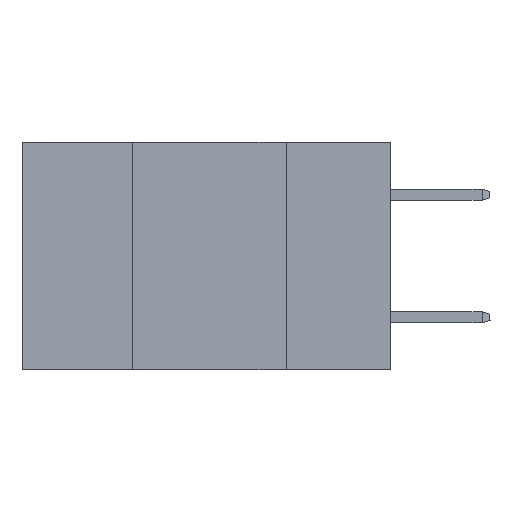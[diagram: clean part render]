
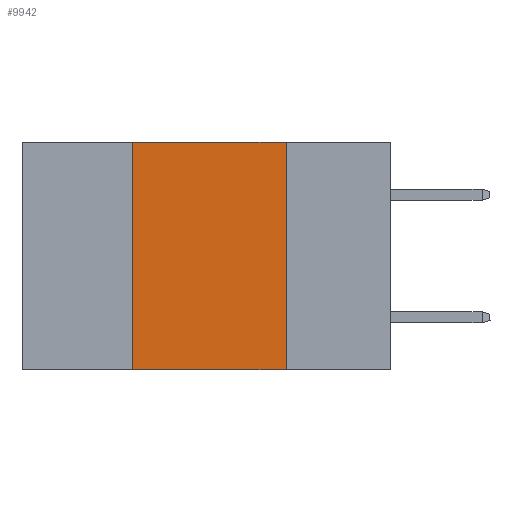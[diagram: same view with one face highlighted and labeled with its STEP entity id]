
A CAD part, left-side view. The second image highlights one B-rep face of the part: STEP entity #9942.
In plain terms, the highlighted planar face has unit normal (-1, 0, 0).
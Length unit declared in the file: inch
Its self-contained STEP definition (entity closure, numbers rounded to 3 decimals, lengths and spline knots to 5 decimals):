
#771 = VERTEX_POINT ( 'NONE', #9905 ) ;
#997 = DIRECTION ( 'NONE',  ( 0., -1., 0. ) ) ;
#1501 = LINE ( 'NONE', #6067, #5940 ) ;
#2105 = VECTOR ( 'NONE', #5797, 39.37008 ) ;
#3709 = CARTESIAN_POINT ( 'NONE',  ( 0., 0.6, 0. ) ) ;
#3870 = LINE ( 'NONE', #14159, #14674 ) ;
#3952 = EDGE_CURVE ( 'NONE', #10515, #14036, #3870, .T. ) ;
#3981 = DIRECTION ( 'NONE',  ( 0., 0., 1. ) ) ;
#4027 = CARTESIAN_POINT ( 'NONE',  ( 0., 0.17, -0.37 ) ) ;
#4431 = CARTESIAN_POINT ( 'NONE',  ( 0., 0.6, -0.37 ) ) ;
#4781 = EDGE_LOOP ( 'NONE', ( #12179, #7769, #14538, #7964 ) ) ;
#4907 = EDGE_CURVE ( 'NONE', #771, #14106, #1501, .T. ) ;
#4952 = CARTESIAN_POINT ( 'NONE',  ( 0., 0.6, 0. ) ) ;
#5797 = DIRECTION ( 'NONE',  ( 0., -1., 0. ) ) ;
#5940 = VECTOR ( 'NONE', #3981, 39.37008 ) ;
#6067 = CARTESIAN_POINT ( 'NONE',  ( 0., 0.42, 0. ) ) ;
#6235 = DIRECTION ( 'NONE',  ( 1., 0., 0. ) ) ;
#7500 = PLANE ( 'NONE',  #9769 ) ;
#7769 = ORIENTED_EDGE ( 'NONE', *, *, #8009, .F. ) ;
#7848 = LINE ( 'NONE', #4431, #9333 ) ;
#7964 = ORIENTED_EDGE ( 'NONE', *, *, #11619, .T. ) ;
#8009 = EDGE_CURVE ( 'NONE', #14106, #10515, #13785, .T. ) ;
#8406 = DIRECTION ( 'NONE',  ( 0., 0., -1. ) ) ;
#9333 = VECTOR ( 'NONE', #997, 39.37008 ) ;
#9769 = AXIS2_PLACEMENT_3D ( 'NONE', #4952, #6235, #14281 ) ;
#9905 = CARTESIAN_POINT ( 'NONE',  ( 0., 0.42, -0.37 ) ) ;
#9942 = ADVANCED_FACE ( 'NONE', ( #12944 ), #7500, .F. ) ;
#10011 = CARTESIAN_POINT ( 'NONE',  ( 0., 0.17, 0. ) ) ;
#10515 = VERTEX_POINT ( 'NONE', #10011 ) ;
#11619 = EDGE_CURVE ( 'NONE', #771, #14036, #7848, .T. ) ;
#12179 = ORIENTED_EDGE ( 'NONE', *, *, #3952, .F. ) ;
#12944 = FACE_OUTER_BOUND ( 'NONE', #4781, .T. ) ;
#13116 = CARTESIAN_POINT ( 'NONE',  ( 0., 0.42, 0. ) ) ;
#13785 = LINE ( 'NONE', #3709, #2105 ) ;
#14036 = VERTEX_POINT ( 'NONE', #4027 ) ;
#14106 = VERTEX_POINT ( 'NONE', #13116 ) ;
#14159 = CARTESIAN_POINT ( 'NONE',  ( 0., 0.17, 0. ) ) ;
#14281 = DIRECTION ( 'NONE',  ( 0., 0., -1. ) ) ;
#14538 = ORIENTED_EDGE ( 'NONE', *, *, #4907, .F. ) ;
#14674 = VECTOR ( 'NONE', #8406, 39.37008 ) ;
